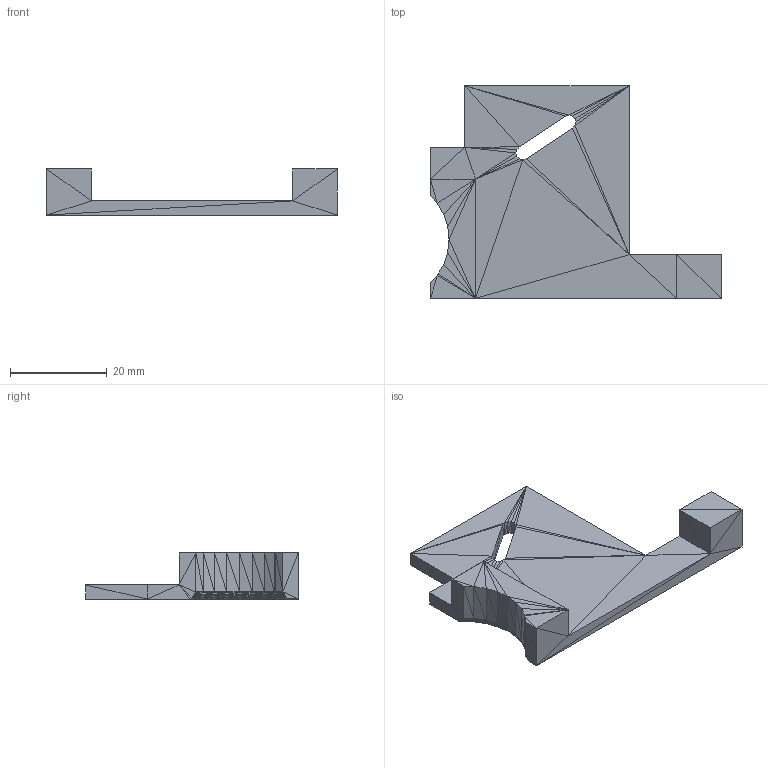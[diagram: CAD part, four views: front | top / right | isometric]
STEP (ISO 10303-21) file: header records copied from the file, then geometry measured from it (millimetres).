
FILE_DESCRIPTION(('FreeCAD Model'),'2;1');
FILE_NAME('Open CASCADE Shape Model','2021-09-30T11:59:09',('Author'),( ''),'Open CASCADE STEP processor 7.4','FreeCAD','Unknown');
FILE_SCHEMA(('AUTOMOTIVE_DESIGN { 1 0 10303 214 1 1 1 1 }'));
Length unit declared in the file: millimetre
Products named in the file (1): Trigger_Right001_(Solid)
Bounding box: 60.07 x 43.94 x 9.53 mm (x, y, z)
Volume: 6996.9 mm3; surface area: 4996.1 mm2
Topology: 1 solids, 1 shells, 332 faces, 498 edges, 166 vertices
Faces by surface type: plane 332
Entity records: 12480 total; most frequent: CARTESIAN_POINT 2491, DIRECTION 1662, ORIENTED_EDGE 996, LINE 996, VECTOR 996, PCURVE 996, DEFINITIONAL_REPRESENTATION 996, EDGE_CURVE 498
